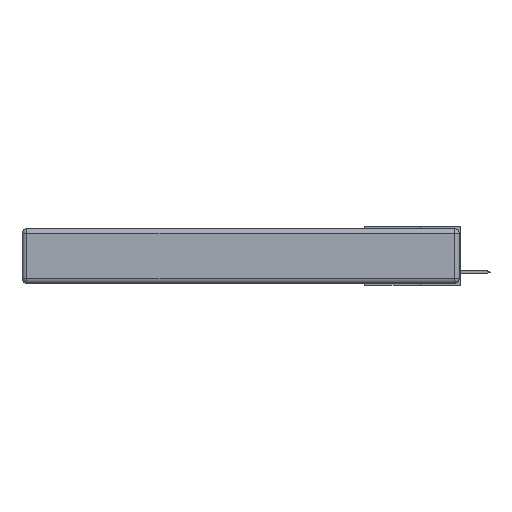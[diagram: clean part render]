
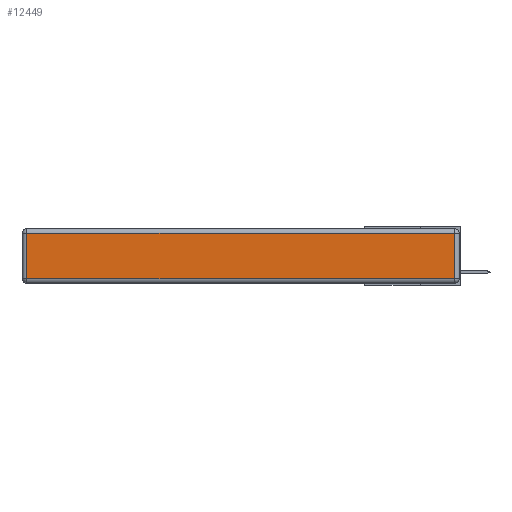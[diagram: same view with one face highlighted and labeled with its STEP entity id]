
A CAD part, left-side view. The second image highlights one B-rep face of the part: STEP entity #12449.
In plain terms, the highlighted planar face has unit normal (-1, 0, 0).
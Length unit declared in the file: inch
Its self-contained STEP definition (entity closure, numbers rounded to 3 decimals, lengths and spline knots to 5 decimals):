
#246 = CARTESIAN_POINT ( 'NONE',  ( 0., 0.03, -0.03 ) ) ;
#266 = ORIENTED_EDGE ( 'NONE', *, *, #12761, .T. ) ;
#877 = DIRECTION ( 'NONE',  ( 0., -1., 0. ) ) ;
#936 = VERTEX_POINT ( 'NONE', #13139 ) ;
#1109 = VECTOR ( 'NONE', #12100, 39.37008 ) ;
#1879 = EDGE_CURVE ( 'NONE', #936, #5856, #8381, .T. ) ;
#3389 = LINE ( 'NONE', #4181, #6882 ) ;
#4042 = LINE ( 'NONE', #5423, #1109 ) ;
#4181 = CARTESIAN_POINT ( 'NONE',  ( 0., 0., -0.313 ) ) ;
#4401 = CARTESIAN_POINT ( 'NONE',  ( 0., 0., -0.343 ) ) ;
#4427 = ORIENTED_EDGE ( 'NONE', *, *, #7934, .T. ) ;
#4448 = DIRECTION ( 'NONE',  ( 0., 0., -1. ) ) ;
#4502 = CARTESIAN_POINT ( 'NONE',  ( 0., 2.72, -0.03 ) ) ;
#5423 = CARTESIAN_POINT ( 'NONE',  ( 0., 2.75, -0.03 ) ) ;
#5818 = ORIENTED_EDGE ( 'NONE', *, *, #1879, .T. ) ;
#5856 = VERTEX_POINT ( 'NONE', #246 ) ;
#6154 = ORIENTED_EDGE ( 'NONE', *, *, #9071, .T. ) ;
#6501 = DIRECTION ( 'NONE',  ( -1., 0., 0. ) ) ;
#6882 = VECTOR ( 'NONE', #877, 39.37008 ) ;
#7325 = LINE ( 'NONE', #9912, #9951 ) ;
#7656 = VERTEX_POINT ( 'NONE', #4502 ) ;
#7822 = DIRECTION ( 'NONE',  ( 0., 0., 1. ) ) ;
#7934 = EDGE_CURVE ( 'NONE', #5856, #7656, #4042, .T. ) ;
#8105 = FACE_OUTER_BOUND ( 'NONE', #12273, .T. ) ;
#8381 = LINE ( 'NONE', #10780, #13315 ) ;
#9071 = EDGE_CURVE ( 'NONE', #7656, #11578, #7325, .T. ) ;
#9636 = AXIS2_PLACEMENT_3D ( 'NONE', #4401, #6501, #7822 ) ;
#9912 = CARTESIAN_POINT ( 'NONE',  ( 0., 2.72, -0.343 ) ) ;
#9951 = VECTOR ( 'NONE', #4448, 39.37008 ) ;
#10780 = CARTESIAN_POINT ( 'NONE',  ( 0., 0.03, -0.343 ) ) ;
#11578 = VERTEX_POINT ( 'NONE', #12388 ) ;
#12100 = DIRECTION ( 'NONE',  ( 0., 1., 0. ) ) ;
#12273 = EDGE_LOOP ( 'NONE', ( #266, #5818, #4427, #6154 ) ) ;
#12388 = CARTESIAN_POINT ( 'NONE',  ( 0., 2.72, -0.313 ) ) ;
#12449 = ADVANCED_FACE ( 'NONE', ( #8105 ), #13189, .T. ) ;
#12761 = EDGE_CURVE ( 'NONE', #11578, #936, #3389, .T. ) ;
#13139 = CARTESIAN_POINT ( 'NONE',  ( 0., 0.03, -0.313 ) ) ;
#13189 = PLANE ( 'NONE',  #9636 ) ;
#13315 = VECTOR ( 'NONE', #14348, 39.37008 ) ;
#14348 = DIRECTION ( 'NONE',  ( 0., 0., 1. ) ) ;
